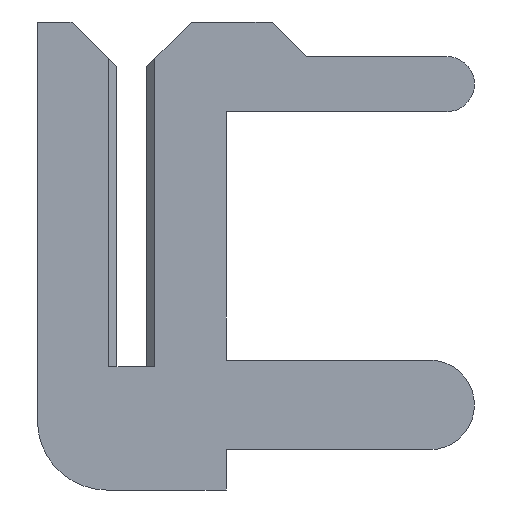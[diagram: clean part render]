
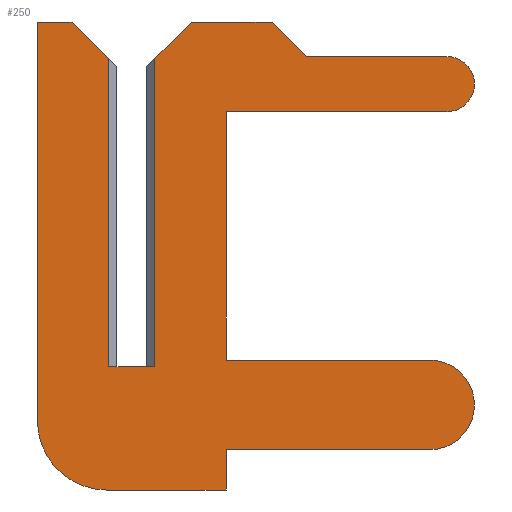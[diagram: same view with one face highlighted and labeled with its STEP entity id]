
A CAD part, left-side view. The second image highlights one B-rep face of the part: STEP entity #250.
In plain terms, the highlighted planar face has unit normal (-1, 0, 0).
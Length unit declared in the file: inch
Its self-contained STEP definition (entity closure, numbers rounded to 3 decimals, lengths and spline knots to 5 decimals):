
#2 = CARTESIAN_POINT ( 'NONE',  ( -0.01, 0.026, 0.15 ) ) ;
#8 = ORIENTED_EDGE ( 'NONE', *, *, #296, .F. ) ;
#9 = CARTESIAN_POINT ( 'NONE',  ( -0.01, -0.041, 0.003 ) ) ;
#26 = CARTESIAN_POINT ( 'NONE',  ( -0.01, 0.011, -0.0535 ) ) ;
#28 = DIRECTION ( 'NONE',  ( 0., 1., 0. ) ) ;
#39 = CARTESIAN_POINT ( 'NONE',  ( -0.01, -0.1295, -0.0165 ) ) ;
#42 = ORIENTED_EDGE ( 'NONE', *, *, #1057, .F. ) ;
#51 = CARTESIAN_POINT ( 'NONE',  ( -0.01, -0.137, 0.135 ) ) ;
#57 = VERTEX_POINT ( 'NONE', #196 ) ;
#58 = LINE ( 'NONE', #247, #461 ) ;
#67 = DIRECTION ( 'NONE',  ( 0., -1., 0. ) ) ;
#70 = VERTEX_POINT ( 'NONE', #703 ) ;
#72 = VERTEX_POINT ( 'NONE', #359 ) ;
#93 = DIRECTION ( 'NONE',  ( 0., 0., 1. ) ) ;
#110 = DIRECTION ( 'NONE',  ( 0., 0., -1. ) ) ;
#116 = CARTESIAN_POINT ( 'NONE',  ( -0.01, 0.0065, 0.1305 ) ) ;
#129 = ORIENTED_EDGE ( 'NONE', *, *, #482, .T. ) ;
#130 = VECTOR ( 'NONE', #341, 39.37008 ) ;
#135 = DIRECTION ( 'NONE',  ( 0., -0.707, -0.707 ) ) ;
#141 = VECTOR ( 'NONE', #521, 39.37008 ) ;
#152 = CARTESIAN_POINT ( 'NONE',  ( -0.01, -0.1295, 0.003 ) ) ;
#153 = VECTOR ( 'NONE', #592, 39.37008 ) ;
#155 = VECTOR ( 'NONE', #318, 39.37008 ) ;
#178 = DIRECTION ( 'NONE',  ( 0., 0., -1. ) ) ;
#185 = ORIENTED_EDGE ( 'NONE', *, *, #385, .F. ) ;
#196 = CARTESIAN_POINT ( 'NONE',  ( -0.01, -0.1295, -0.036 ) ) ;
#204 = VERTEX_POINT ( 'NONE', #930 ) ;
#206 = LINE ( 'NONE', #1037, #865 ) ;
#208 = ORIENTED_EDGE ( 'NONE', *, *, #625, .F. ) ;
#223 = DIRECTION ( 'NONE',  ( 0., 0., 1. ) ) ;
#226 = CARTESIAN_POINT ( 'NONE',  ( -0.01, 0.01, 0. ) ) ;
#247 = CARTESIAN_POINT ( 'NONE',  ( -0.01, -0.076, 0.135 ) ) ;
#248 = EDGE_CURVE ( 'NONE', #916, #938, #323, .T. ) ;
#250 = ADVANCED_FACE ( 'NONE', ( #712 ), #847, .T. ) ;
#252 = DIRECTION ( 'NONE',  ( 0., 0., 1. ) ) ;
#291 = LINE ( 'NONE', #26, #1036 ) ;
#296 = EDGE_CURVE ( 'NONE', #537, #1059, #677, .T. ) ;
#307 = DIRECTION ( 'NONE',  ( 0., 0., 1. ) ) ;
#318 = DIRECTION ( 'NONE',  ( 0., -1., 0. ) ) ;
#323 = LINE ( 'NONE', #941, #536 ) ;
#330 = CARTESIAN_POINT ( 'NONE',  ( -0.01, 0.011, -0.0235 ) ) ;
#339 = LINE ( 'NONE', #927, #882 ) ;
#341 = DIRECTION ( 'NONE',  ( 0., 1., 0. ) ) ;
#342 = CARTESIAN_POINT ( 'NONE',  ( -0.01, -0.041, -0.0535 ) ) ;
#344 = EDGE_CURVE ( 'NONE', #1095, #1010, #725, .T. ) ;
#359 = CARTESIAN_POINT ( 'NONE',  ( -0.01, -0.041, -0.036 ) ) ;
#360 = CARTESIAN_POINT ( 'NONE',  ( -0.01, -0.076, 0.135 ) ) ;
#371 = EDGE_CURVE ( 'NONE', #681, #611, #291, .T. ) ;
#374 = ORIENTED_EDGE ( 'NONE', *, *, #505, .F. ) ;
#375 = CARTESIAN_POINT ( 'NONE',  ( -0.01, -0.01, 0.134 ) ) ;
#381 = CIRCLE ( 'NONE', #472, 0.0195 ) ;
#384 = VERTEX_POINT ( 'NONE', #226 ) ;
#385 = EDGE_CURVE ( 'NONE', #938, #57, #381, .T. ) ;
#409 = VERTEX_POINT ( 'NONE', #649 ) ;
#411 = DIRECTION ( 'NONE',  ( 0., -0.707, 0.707 ) ) ;
#419 = ORIENTED_EDGE ( 'NONE', *, *, #371, .F. ) ;
#424 = EDGE_CURVE ( 'NONE', #616, #70, #848, .T. ) ;
#429 = CARTESIAN_POINT ( 'NONE',  ( -0.01, -0.137, 0.111 ) ) ;
#434 = VECTOR ( 'NONE', #683, 39.37008 ) ;
#437 = CARTESIAN_POINT ( 'NONE',  ( -0.01, 0.041, 0.15 ) ) ;
#461 = VECTOR ( 'NONE', #513, 39.37008 ) ;
#472 = AXIS2_PLACEMENT_3D ( 'NONE', #39, #659, #223 ) ;
#482 = EDGE_CURVE ( 'NONE', #384, #70, #206, .T. ) ;
#500 = ORIENTED_EDGE ( 'NONE', *, *, #424, .F. ) ;
#505 = EDGE_CURVE ( 'NONE', #582, #616, #612, .T. ) ;
#513 = DIRECTION ( 'NONE',  ( 0., -0.707, -0.707 ) ) ;
#516 = DIRECTION ( 'NONE',  ( 0., 1., 0. ) ) ;
#520 = CIRCLE ( 'NONE', #1021, 0.012 ) ;
#521 = DIRECTION ( 'NONE',  ( 0., -1., 0. ) ) ;
#526 = CARTESIAN_POINT ( 'NONE',  ( -0.01, 0.0065, 0. ) ) ;
#536 = VECTOR ( 'NONE', #67, 39.37008 ) ;
#537 = VERTEX_POINT ( 'NONE', #360 ) ;
#544 = DIRECTION ( 'NONE',  ( 1., 0., 0. ) ) ;
#549 = ORIENTED_EDGE ( 'NONE', *, *, #1078, .F. ) ;
#550 = VECTOR ( 'NONE', #135, 39.37008 ) ;
#551 = VECTOR ( 'NONE', #252, 39.37008 ) ;
#566 = AXIS2_PLACEMENT_3D ( 'NONE', #1056, #544, #720 ) ;
#567 = ORIENTED_EDGE ( 'NONE', *, *, #344, .F. ) ;
#582 = VERTEX_POINT ( 'NONE', #614 ) ;
#588 = CARTESIAN_POINT ( 'NONE',  ( -0.01, -0.137, 0.123 ) ) ;
#592 = DIRECTION ( 'NONE',  ( 0., -1., 0. ) ) ;
#593 = EDGE_CURVE ( 'NONE', #72, #681, #647, .T. ) ;
#594 = ORIENTED_EDGE ( 'NONE', *, *, #248, .F. ) ;
#601 = DIRECTION ( 'NONE',  ( 0., 0., -1. ) ) ;
#602 = CARTESIAN_POINT ( 'NONE',  ( -0.01, -0.137, 0.135 ) ) ;
#611 = VERTEX_POINT ( 'NONE', #873 ) ;
#612 = LINE ( 'NONE', #2, #141 ) ;
#614 = CARTESIAN_POINT ( 'NONE',  ( -0.01, 0.041, 0.15 ) ) ;
#616 = VERTEX_POINT ( 'NONE', #1042 ) ;
#618 = EDGE_CURVE ( 'NONE', #1035, #582, #1121, .T. ) ;
#625 = EDGE_CURVE ( 'NONE', #611, #1035, #867, .T. ) ;
#632 = LINE ( 'NONE', #854, #977 ) ;
#644 = ORIENTED_EDGE ( 'NONE', *, *, #754, .F. ) ;
#647 = LINE ( 'NONE', #342, #897 ) ;
#649 = CARTESIAN_POINT ( 'NONE',  ( -0.01, -0.01, 0. ) ) ;
#659 = DIRECTION ( 'NONE',  ( 1., 0., 0. ) ) ;
#677 = LINE ( 'NONE', #51, #155 ) ;
#681 = VERTEX_POINT ( 'NONE', #1048 ) ;
#683 = DIRECTION ( 'NONE',  ( 0., -1., 0. ) ) ;
#696 = VERTEX_POINT ( 'NONE', #375 ) ;
#703 = CARTESIAN_POINT ( 'NONE',  ( -0.01, 0.01, 0.134 ) ) ;
#712 = FACE_OUTER_BOUND ( 'NONE', #1052, .T. ) ;
#720 = DIRECTION ( 'NONE',  ( 0., 0., 1. ) ) ;
#725 = LINE ( 'NONE', #857, #130 ) ;
#734 = VERTEX_POINT ( 'NONE', #889 ) ;
#736 = EDGE_CURVE ( 'NONE', #1010, #916, #950, .T. ) ;
#754 = EDGE_CURVE ( 'NONE', #57, #72, #339, .T. ) ;
#773 = CARTESIAN_POINT ( 'NONE',  ( -0.01, -0.041, 0.111 ) ) ;
#792 = ORIENTED_EDGE ( 'NONE', *, *, #891, .F. ) ;
#799 = CARTESIAN_POINT ( 'NONE',  ( -0.01, -0.041, 0.003 ) ) ;
#806 = EDGE_CURVE ( 'NONE', #696, #409, #632, .T. ) ;
#823 = EDGE_CURVE ( 'NONE', #1059, #1095, #520, .T. ) ;
#826 = LINE ( 'NONE', #1029, #434 ) ;
#830 = AXIS2_PLACEMENT_3D ( 'NONE', #330, #898, #307 ) ;
#843 = DIRECTION ( 'NONE',  ( 1., 0., 0. ) ) ;
#847 = PLANE ( 'NONE',  #830 ) ;
#848 = LINE ( 'NONE', #116, #550 ) ;
#853 = ORIENTED_EDGE ( 'NONE', *, *, #593, .F. ) ;
#854 = CARTESIAN_POINT ( 'NONE',  ( -0.01, -0.01, 0.15 ) ) ;
#857 = CARTESIAN_POINT ( 'NONE',  ( -0.01, -0.041, 0.111 ) ) ;
#864 = ORIENTED_EDGE ( 'NONE', *, *, #823, .F. ) ;
#865 = VECTOR ( 'NONE', #93, 39.37008 ) ;
#867 = CIRCLE ( 'NONE', #566, 0.03 ) ;
#873 = CARTESIAN_POINT ( 'NONE',  ( -0.01, 0.011, -0.0535 ) ) ;
#882 = VECTOR ( 'NONE', #516, 39.37008 ) ;
#889 = CARTESIAN_POINT ( 'NONE',  ( -0.01, -0.026, 0.15 ) ) ;
#891 = EDGE_CURVE ( 'NONE', #696, #734, #1093, .T. ) ;
#897 = VECTOR ( 'NONE', #178, 39.37008 ) ;
#898 = DIRECTION ( 'NONE',  ( -1., 0., 0. ) ) ;
#907 = ORIENTED_EDGE ( 'NONE', *, *, #618, .F. ) ;
#916 = VERTEX_POINT ( 'NONE', #799 ) ;
#924 = EDGE_CURVE ( 'NONE', #734, #204, #826, .T. ) ;
#927 = CARTESIAN_POINT ( 'NONE',  ( -0.01, -0.041, -0.036 ) ) ;
#930 = CARTESIAN_POINT ( 'NONE',  ( -0.01, -0.061, 0.15 ) ) ;
#934 = ORIENTED_EDGE ( 'NONE', *, *, #736, .F. ) ;
#938 = VERTEX_POINT ( 'NONE', #152 ) ;
#941 = CARTESIAN_POINT ( 'NONE',  ( -0.01, -0.1295, 0.003 ) ) ;
#942 = CARTESIAN_POINT ( 'NONE',  ( -0.01, -0.0065, 0.1305 ) ) ;
#950 = LINE ( 'NONE', #9, #1040 ) ;
#977 = VECTOR ( 'NONE', #601, 39.37008 ) ;
#987 = LINE ( 'NONE', #526, #153 ) ;
#1010 = VERTEX_POINT ( 'NONE', #773 ) ;
#1019 = DIRECTION ( 'NONE',  ( 0., 0., 1. ) ) ;
#1021 = AXIS2_PLACEMENT_3D ( 'NONE', #588, #843, #1019 ) ;
#1029 = CARTESIAN_POINT ( 'NONE',  ( -0.01, -0.026, 0.15 ) ) ;
#1032 = CARTESIAN_POINT ( 'NONE',  ( -0.01, 0.041, -0.0235 ) ) ;
#1035 = VERTEX_POINT ( 'NONE', #1032 ) ;
#1036 = VECTOR ( 'NONE', #28, 39.37008 ) ;
#1037 = CARTESIAN_POINT ( 'NONE',  ( -0.01, 0.01, -0.0235 ) ) ;
#1040 = VECTOR ( 'NONE', #110, 39.37008 ) ;
#1042 = CARTESIAN_POINT ( 'NONE',  ( -0.01, 0.026, 0.15 ) ) ;
#1048 = CARTESIAN_POINT ( 'NONE',  ( -0.01, -0.041, -0.0535 ) ) ;
#1052 = EDGE_LOOP ( 'NONE', ( #792, #1091, #549, #129, #500, #374, #907, #208, #419, #853, #644, #185, #594, #934, #567, #864, #8, #42, #1103 ) ) ;
#1056 = CARTESIAN_POINT ( 'NONE',  ( -0.01, 0.011, -0.0235 ) ) ;
#1057 = EDGE_CURVE ( 'NONE', #204, #537, #58, .T. ) ;
#1059 = VERTEX_POINT ( 'NONE', #602 ) ;
#1070 = VECTOR ( 'NONE', #411, 39.37008 ) ;
#1078 = EDGE_CURVE ( 'NONE', #384, #409, #987, .T. ) ;
#1091 = ORIENTED_EDGE ( 'NONE', *, *, #806, .T. ) ;
#1093 = LINE ( 'NONE', #942, #1070 ) ;
#1095 = VERTEX_POINT ( 'NONE', #429 ) ;
#1103 = ORIENTED_EDGE ( 'NONE', *, *, #924, .F. ) ;
#1121 = LINE ( 'NONE', #437, #551 ) ;
